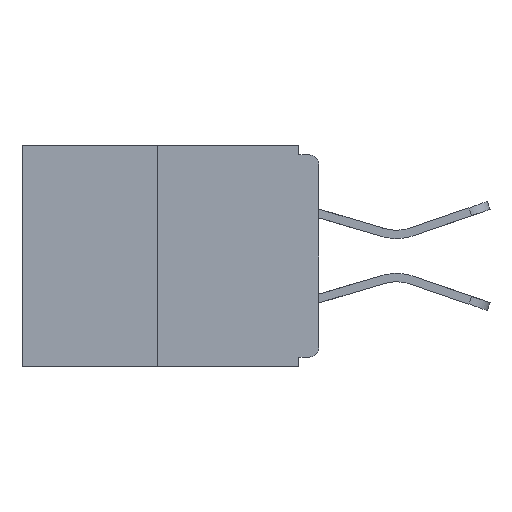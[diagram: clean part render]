
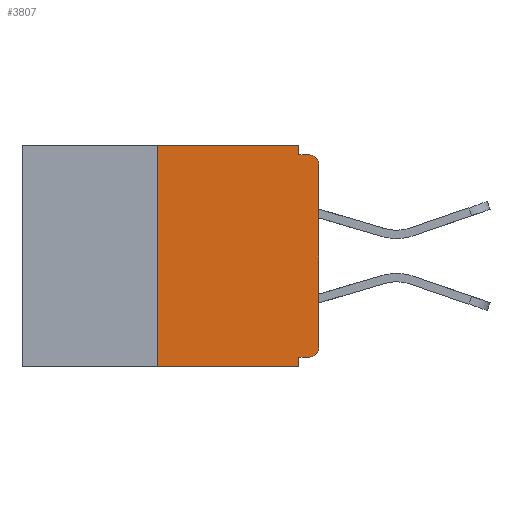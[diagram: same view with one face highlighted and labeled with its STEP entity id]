
A CAD part, left-side view. The second image highlights one B-rep face of the part: STEP entity #3807.
In plain terms, the highlighted planar face has unit normal (-1, 0, 0).
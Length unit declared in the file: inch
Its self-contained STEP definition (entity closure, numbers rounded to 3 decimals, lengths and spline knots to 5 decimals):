
#24 = ORIENTED_EDGE ( 'NONE', *, *, #5586, .T. ) ;
#565 = CARTESIAN_POINT ( 'NONE',  ( 0., 0., -0.313 ) ) ;
#757 = EDGE_CURVE ( 'NONE', #2468, #1881, #5218, .T. ) ;
#805 = VERTEX_POINT ( 'NONE', #8623 ) ;
#1298 = EDGE_LOOP ( 'NONE', ( #7392, #13916, #2100, #5105, #14307, #7311, #24, #3475, #2193, #6791 ) ) ;
#1338 = LINE ( 'NONE', #11217, #1490 ) ;
#1417 = CARTESIAN_POINT ( 'NONE',  ( 0., 0.031, 0. ) ) ;
#1490 = VECTOR ( 'NONE', #12365, 39.37008 ) ;
#1708 = DIRECTION ( 'NONE',  ( 0., -1., 0. ) ) ;
#1881 = VERTEX_POINT ( 'NONE', #14434 ) ;
#1985 = VECTOR ( 'NONE', #13597, 39.37008 ) ;
#2100 = ORIENTED_EDGE ( 'NONE', *, *, #7683, .T. ) ;
#2157 = VECTOR ( 'NONE', #1708, 39.37008 ) ;
#2193 = ORIENTED_EDGE ( 'NONE', *, *, #15510, .F. ) ;
#2468 = VERTEX_POINT ( 'NONE', #4864 ) ;
#2493 = CARTESIAN_POINT ( 'NONE',  ( 0., 0.031, -0.343 ) ) ;
#2533 = VERTEX_POINT ( 'NONE', #7642 ) ;
#2680 = LINE ( 'NONE', #1417, #11873 ) ;
#2808 = CIRCLE ( 'NONE', #13346, 0.015 ) ;
#2869 = CARTESIAN_POINT ( 'NONE',  ( 0., 0.46, 0. ) ) ;
#3446 = LINE ( 'NONE', #4653, #6645 ) ;
#3475 = ORIENTED_EDGE ( 'NONE', *, *, #11906, .T. ) ;
#3507 = VERTEX_POINT ( 'NONE', #12417 ) ;
#3599 = EDGE_CURVE ( 'NONE', #2533, #4226, #14009, .T. ) ;
#3807 = ADVANCED_FACE ( 'NONE', ( #11157 ), #4611, .F. ) ;
#4226 = VERTEX_POINT ( 'NONE', #7468 ) ;
#4611 = PLANE ( 'NONE',  #9305 ) ;
#4653 = CARTESIAN_POINT ( 'NONE',  ( 0., 0., -0.015 ) ) ;
#4745 = CARTESIAN_POINT ( 'NONE',  ( 0., 0., -0.328 ) ) ;
#4789 = CARTESIAN_POINT ( 'NONE',  ( 0., 0.015, -0.03 ) ) ;
#4864 = CARTESIAN_POINT ( 'NONE',  ( 0., 0.031, -0.328 ) ) ;
#5000 = VERTEX_POINT ( 'NONE', #565 ) ;
#5036 = CARTESIAN_POINT ( 'NONE',  ( 0., 0.031, -0.015 ) ) ;
#5105 = ORIENTED_EDGE ( 'NONE', *, *, #757, .F. ) ;
#5145 = DIRECTION ( 'NONE',  ( 0., 0., -1. ) ) ;
#5218 = LINE ( 'NONE', #2493, #11233 ) ;
#5586 = EDGE_CURVE ( 'NONE', #5000, #9073, #1338, .T. ) ;
#5668 = DIRECTION ( 'NONE',  ( 1., 0., 0. ) ) ;
#6093 = CIRCLE ( 'NONE', #10686, 0.015 ) ;
#6221 = EDGE_CURVE ( 'NONE', #3507, #2468, #10515, .T. ) ;
#6645 = VECTOR ( 'NONE', #14320, 39.37008 ) ;
#6779 = VERTEX_POINT ( 'NONE', #5036 ) ;
#6791 = ORIENTED_EDGE ( 'NONE', *, *, #10368, .F. ) ;
#6821 = DIRECTION ( 'NONE',  ( 0., 0., -1. ) ) ;
#6887 = DIRECTION ( 'NONE',  ( -1., 0., 0. ) ) ;
#7136 = CARTESIAN_POINT ( 'NONE',  ( 0., 0., -0.03 ) ) ;
#7311 = ORIENTED_EDGE ( 'NONE', *, *, #9042, .T. ) ;
#7315 = DIRECTION ( 'NONE',  ( 0., -1., 0. ) ) ;
#7332 = VECTOR ( 'NONE', #13111, 39.37008 ) ;
#7392 = ORIENTED_EDGE ( 'NONE', *, *, #15362, .F. ) ;
#7468 = CARTESIAN_POINT ( 'NONE',  ( 0., 0.25, 0. ) ) ;
#7642 = CARTESIAN_POINT ( 'NONE',  ( 0., 0.25, -0.343 ) ) ;
#7649 = VECTOR ( 'NONE', #7315, 39.37008 ) ;
#7683 = EDGE_CURVE ( 'NONE', #2533, #1881, #14788, .T. ) ;
#8623 = CARTESIAN_POINT ( 'NONE',  ( 0., 0.015, -0.015 ) ) ;
#9042 = EDGE_CURVE ( 'NONE', #3507, #5000, #6093, .T. ) ;
#9073 = VERTEX_POINT ( 'NONE', #7136 ) ;
#9305 = AXIS2_PLACEMENT_3D ( 'NONE', #15271, #5668, #6821 ) ;
#9827 = DIRECTION ( 'NONE',  ( 0., 0., -1. ) ) ;
#10368 = EDGE_CURVE ( 'NONE', #11230, #6779, #2680, .T. ) ;
#10515 = LINE ( 'NONE', #4745, #7332 ) ;
#10649 = CARTESIAN_POINT ( 'NONE',  ( 0., 0.015, -0.313 ) ) ;
#10686 = AXIS2_PLACEMENT_3D ( 'NONE', #10649, #6887, #11905 ) ;
#11157 = FACE_OUTER_BOUND ( 'NONE', #1298, .T. ) ;
#11217 = CARTESIAN_POINT ( 'NONE',  ( 0., 0., 0. ) ) ;
#11230 = VERTEX_POINT ( 'NONE', #12788 ) ;
#11233 = VECTOR ( 'NONE', #9827, 39.37008 ) ;
#11711 = LINE ( 'NONE', #2869, #2157 ) ;
#11873 = VECTOR ( 'NONE', #13354, 39.37008 ) ;
#11905 = DIRECTION ( 'NONE',  ( 0., 0., -1. ) ) ;
#11906 = EDGE_CURVE ( 'NONE', #9073, #805, #2808, .T. ) ;
#12287 = DIRECTION ( 'NONE',  ( -1., 0., 0. ) ) ;
#12365 = DIRECTION ( 'NONE',  ( 0., 0., 1. ) ) ;
#12417 = CARTESIAN_POINT ( 'NONE',  ( 0., 0.015, -0.328 ) ) ;
#12788 = CARTESIAN_POINT ( 'NONE',  ( 0., 0.031, 0. ) ) ;
#13111 = DIRECTION ( 'NONE',  ( 0., 1., 0. ) ) ;
#13201 = CARTESIAN_POINT ( 'NONE',  ( 0., 0.46, -0.343 ) ) ;
#13346 = AXIS2_PLACEMENT_3D ( 'NONE', #4789, #12287, #5145 ) ;
#13354 = DIRECTION ( 'NONE',  ( 0., 0., -1. ) ) ;
#13544 = CARTESIAN_POINT ( 'NONE',  ( 0., 0.25, 0. ) ) ;
#13597 = DIRECTION ( 'NONE',  ( 0., 0., 1. ) ) ;
#13916 = ORIENTED_EDGE ( 'NONE', *, *, #3599, .F. ) ;
#14009 = LINE ( 'NONE', #13544, #1985 ) ;
#14307 = ORIENTED_EDGE ( 'NONE', *, *, #6221, .F. ) ;
#14320 = DIRECTION ( 'NONE',  ( 0., -1., 0. ) ) ;
#14434 = CARTESIAN_POINT ( 'NONE',  ( 0., 0.031, -0.343 ) ) ;
#14788 = LINE ( 'NONE', #13201, #7649 ) ;
#15271 = CARTESIAN_POINT ( 'NONE',  ( 0., 0.46, 0. ) ) ;
#15362 = EDGE_CURVE ( 'NONE', #4226, #11230, #11711, .T. ) ;
#15510 = EDGE_CURVE ( 'NONE', #6779, #805, #3446, .T. ) ;
